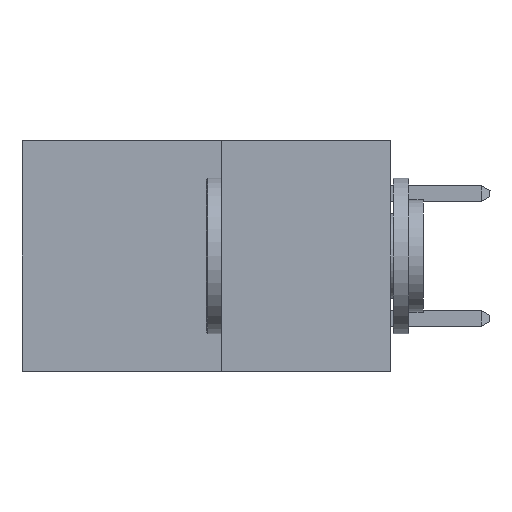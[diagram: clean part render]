
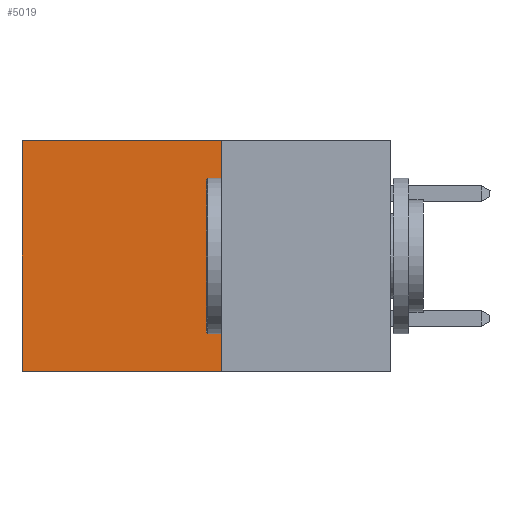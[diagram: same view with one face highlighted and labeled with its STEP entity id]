
A CAD part, left-side view. The second image highlights one B-rep face of the part: STEP entity #5019.
In plain terms, the highlighted planar face has unit normal (-1, 0, 0).
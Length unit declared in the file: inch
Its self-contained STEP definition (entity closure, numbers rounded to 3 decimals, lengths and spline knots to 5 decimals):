
#617 = VECTOR ( 'NONE', #5573, 39.37008 ) ;
#646 = CARTESIAN_POINT ( 'NONE',  ( 0.277, 0.27, -0.37 ) ) ;
#936 = CARTESIAN_POINT ( 'NONE',  ( 0.277, 0.27, -0.37 ) ) ;
#1139 = CARTESIAN_POINT ( 'NONE',  ( 0.277, 0.59, -0.37 ) ) ;
#1231 = DIRECTION ( 'NONE',  ( 0., 0., -1. ) ) ;
#1400 = ORIENTED_EDGE ( 'NONE', *, *, #3919, .T. ) ;
#1539 = EDGE_CURVE ( 'NONE', #4162, #6969, #2640, .T. ) ;
#1869 = ORIENTED_EDGE ( 'NONE', *, *, #2954, .F. ) ;
#1876 = ORIENTED_EDGE ( 'NONE', *, *, #2322, .F. ) ;
#1922 = ORIENTED_EDGE ( 'NONE', *, *, #1539, .T. ) ;
#1984 = LINE ( 'NONE', #6435, #5725 ) ;
#2322 = EDGE_CURVE ( 'NONE', #4162, #9479, #6758, .T. ) ;
#2386 = CARTESIAN_POINT ( 'NONE',  ( 0.277, 0.59, 0. ) ) ;
#2640 = LINE ( 'NONE', #7738, #617 ) ;
#2954 = EDGE_CURVE ( 'NONE', #9479, #3179, #1984, .T. ) ;
#3179 = VERTEX_POINT ( 'NONE', #7020 ) ;
#3244 = EDGE_LOOP ( 'NONE', ( #1400, #1869, #1876, #1922 ) ) ;
#3311 = DIRECTION ( 'NONE',  ( 0., 1., 0. ) ) ;
#3522 = VECTOR ( 'NONE', #1231, 39.37008 ) ;
#3919 = EDGE_CURVE ( 'NONE', #6969, #3179, #9296, .T. ) ;
#4162 = VERTEX_POINT ( 'NONE', #6654 ) ;
#4537 = FACE_OUTER_BOUND ( 'NONE', #3244, .T. ) ;
#4816 = VECTOR ( 'NONE', #9400, 39.37008 ) ;
#5019 = ADVANCED_FACE ( 'NONE', ( #4537 ), #6233, .F. ) ;
#5573 = DIRECTION ( 'NONE',  ( 0., 1., 0. ) ) ;
#5725 = VECTOR ( 'NONE', #3311, 39.37008 ) ;
#5872 = AXIS2_PLACEMENT_3D ( 'NONE', #6301, #6227, #6211 ) ;
#6211 = DIRECTION ( 'NONE',  ( 0., 0., -1. ) ) ;
#6227 = DIRECTION ( 'NONE',  ( 1., 0., 0. ) ) ;
#6233 = PLANE ( 'NONE',  #5872 ) ;
#6301 = CARTESIAN_POINT ( 'NONE',  ( 0.277, 0.27, -0.37 ) ) ;
#6435 = CARTESIAN_POINT ( 'NONE',  ( 0.277, 0.27, -0.37 ) ) ;
#6654 = CARTESIAN_POINT ( 'NONE',  ( 0.277, 0.27, 0. ) ) ;
#6758 = LINE ( 'NONE', #646, #4816 ) ;
#6969 = VERTEX_POINT ( 'NONE', #2386 ) ;
#7020 = CARTESIAN_POINT ( 'NONE',  ( 0.277, 0.59, -0.37 ) ) ;
#7738 = CARTESIAN_POINT ( 'NONE',  ( 0.277, 0.27, 0. ) ) ;
#9296 = LINE ( 'NONE', #1139, #3522 ) ;
#9400 = DIRECTION ( 'NONE',  ( 0., 0., -1. ) ) ;
#9479 = VERTEX_POINT ( 'NONE', #936 ) ;
